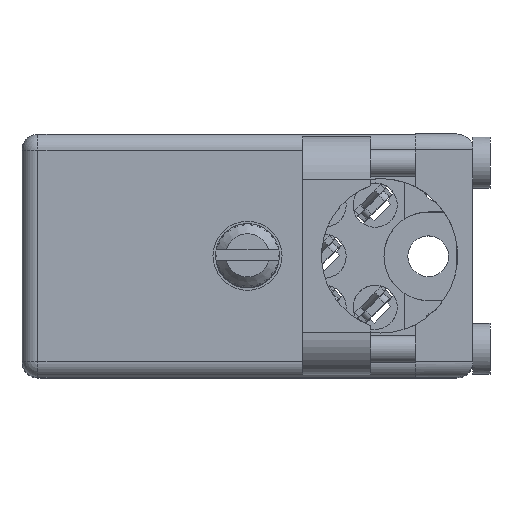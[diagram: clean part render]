
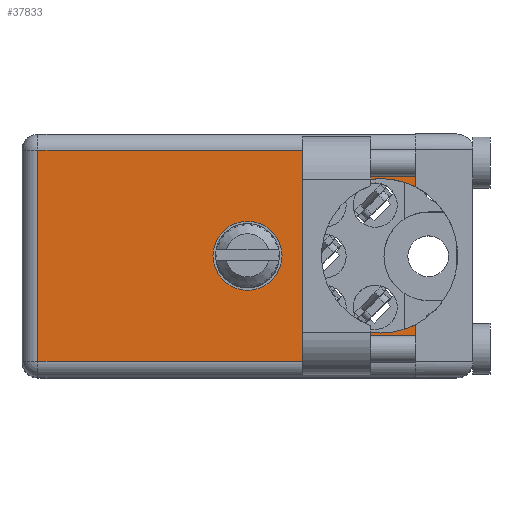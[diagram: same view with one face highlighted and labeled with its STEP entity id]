
A CAD part, top view. The second image highlights one B-rep face of the part: STEP entity #37833.
In plain terms, the highlighted face is planar.
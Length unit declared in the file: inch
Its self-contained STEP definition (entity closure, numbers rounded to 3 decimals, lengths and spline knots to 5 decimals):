
#748 = VERTEX_POINT ( 'NONE', #55095 ) ;
#920 = VERTEX_POINT ( 'NONE', #2474 ) ;
#1799 = CARTESIAN_POINT ( 'NONE',  ( 0.047, 0.906, -0.715 ) ) ;
#2474 = CARTESIAN_POINT ( 'NONE',  ( 0.047, 0.906, -0.668 ) ) ;
#3330 = CARTESIAN_POINT ( 'NONE',  ( 0.6625, 0.906, -0.256 ) ) ;
#3827 = DIRECTION ( 'NONE',  ( 0., 1., 0. ) ) ;
#4999 = DIRECTION ( 'NONE',  ( 0., 0., 1. ) ) ;
#6817 = VERTEX_POINT ( 'NONE', #141544 ) ;
#10199 = AXIS2_PLACEMENT_3D ( 'NONE', #120672, #150699, #94392 ) ;
#11066 = CARTESIAN_POINT ( 'NONE',  ( 0.6625, 0.906, -0.3575 ) ) ;
#19879 = EDGE_LOOP ( 'NONE', ( #52037, #77317, #128347, #160684, #126457, #22712, #62435, #79287 ) ) ;
#22423 = DIRECTION ( 'NONE',  ( 0., 0., 1. ) ) ;
#22712 = ORIENTED_EDGE ( 'NONE', *, *, #29579, .F. ) ;
#25193 = CARTESIAN_POINT ( 'NONE',  ( 1.053, 0.906, -0.5845 ) ) ;
#25256 = VERTEX_POINT ( 'NONE', #25193 ) ;
#26480 = EDGE_CURVE ( 'NONE', #49378, #130904, #122038, .T. ) ;
#27932 = AXIS2_PLACEMENT_3D ( 'NONE', #142008, #84781, #183186 ) ;
#29579 = EDGE_CURVE ( 'NONE', #104759, #6817, #144698, .T. ) ;
#32516 = EDGE_CURVE ( 'NONE', #6817, #130904, #122594, .T. ) ;
#33533 = CIRCLE ( 'NONE', #36447, 0.227 ) ;
#33958 = CIRCLE ( 'NONE', #27932, 0.1015 ) ;
#36340 = DIRECTION ( 'NONE',  ( 0., 0., 1. ) ) ;
#36447 = AXIS2_PLACEMENT_3D ( 'NONE', #36867, #61341, #147645 ) ;
#36867 = CARTESIAN_POINT ( 'NONE',  ( 1.053, 0.906, -0.3575 ) ) ;
#37021 = VECTOR ( 'NONE', #36340, 39.37008 ) ;
#37833 = ADVANCED_FACE ( 'NONE', ( #178746, #107539 ), #176906, .T. ) ;
#39024 = ORIENTED_EDGE ( 'NONE', *, *, #128527, .F. ) ;
#43029 = CIRCLE ( 'NONE', #64029, 0.1015 ) ;
#43716 = CIRCLE ( 'NONE', #163384, 0.227 ) ;
#45681 = EDGE_CURVE ( 'NONE', #25256, #104759, #43716, .T. ) ;
#47749 = DIRECTION ( 'NONE',  ( 0., 0., 1. ) ) ;
#48731 = DIRECTION ( 'NONE',  ( 0., 1., 0. ) ) ;
#48853 = CARTESIAN_POINT ( 'NONE',  ( 0.6625, 0.906, -0.459 ) ) ;
#49378 = VERTEX_POINT ( 'NONE', #103497 ) ;
#52037 = ORIENTED_EDGE ( 'NONE', *, *, #124893, .F. ) ;
#55095 = CARTESIAN_POINT ( 'NONE',  ( 1.155, 0.906, -0.668 ) ) ;
#56113 = DIRECTION ( 'NONE',  ( 0., 1., 0. ) ) ;
#60626 = VECTOR ( 'NONE', #92092, 39.37008 ) ;
#61341 = DIRECTION ( 'NONE',  ( 0., 1., 0. ) ) ;
#62435 = ORIENTED_EDGE ( 'NONE', *, *, #45681, .F. ) ;
#63796 = AXIS2_PLACEMENT_3D ( 'NONE', #151859, #48731, #22423 ) ;
#64029 = AXIS2_PLACEMENT_3D ( 'NONE', #11066, #56113, #125493 ) ;
#66184 = VECTOR ( 'NONE', #102685, 39.37008 ) ;
#71886 = EDGE_LOOP ( 'NONE', ( #39024, #106281 ) ) ;
#72326 = DIRECTION ( 'NONE',  ( 0., 0., 1. ) ) ;
#76281 = LINE ( 'NONE', #159812, #174469 ) ;
#77317 = ORIENTED_EDGE ( 'NONE', *, *, #85751, .T. ) ;
#79287 = ORIENTED_EDGE ( 'NONE', *, *, #99387, .F. ) ;
#84781 = DIRECTION ( 'NONE',  ( 0., 1., 0. ) ) ;
#85751 = EDGE_CURVE ( 'NONE', #748, #920, #172045, .T. ) ;
#92092 = DIRECTION ( 'NONE',  ( 1., 0., 0. ) ) ;
#94003 = CARTESIAN_POINT ( 'NONE',  ( 1.053, 0.906, -0.1305 ) ) ;
#94392 = DIRECTION ( 'NONE',  ( 0., 0., 1. ) ) ;
#97960 = VERTEX_POINT ( 'NONE', #179756 ) ;
#99387 = EDGE_CURVE ( 'NONE', #97960, #25256, #33533, .T. ) ;
#102685 = DIRECTION ( 'NONE',  ( -1., 0., 0. ) ) ;
#103497 = CARTESIAN_POINT ( 'NONE',  ( 0.047, 0.906, -0.047 ) ) ;
#104759 = VERTEX_POINT ( 'NONE', #94003 ) ;
#106281 = ORIENTED_EDGE ( 'NONE', *, *, #108848, .F. ) ;
#107539 = FACE_BOUND ( 'NONE', #71886, .T. ) ;
#108848 = EDGE_CURVE ( 'NONE', #131502, #128381, #43029, .T. ) ;
#120672 = CARTESIAN_POINT ( 'NONE',  ( 0., 0.906, -0.715 ) ) ;
#122038 = LINE ( 'NONE', #167915, #60626 ) ;
#122594 = LINE ( 'NONE', #137593, #37021 ) ;
#124397 = VECTOR ( 'NONE', #47749, 39.37008 ) ;
#124893 = EDGE_CURVE ( 'NONE', #748, #97960, #76281, .T. ) ;
#125493 = DIRECTION ( 'NONE',  ( 0., 0., 1. ) ) ;
#126457 = ORIENTED_EDGE ( 'NONE', *, *, #32516, .F. ) ;
#128347 = ORIENTED_EDGE ( 'NONE', *, *, #141928, .T. ) ;
#128381 = VERTEX_POINT ( 'NONE', #3330 ) ;
#128527 = EDGE_CURVE ( 'NONE', #128381, #131502, #33958, .T. ) ;
#130904 = VERTEX_POINT ( 'NONE', #154246 ) ;
#131409 = CARTESIAN_POINT ( 'NONE',  ( 1.053, 0.906, -0.3575 ) ) ;
#131502 = VERTEX_POINT ( 'NONE', #48853 ) ;
#137593 = CARTESIAN_POINT ( 'NONE',  ( 1.155, 0.906, 0. ) ) ;
#141544 = CARTESIAN_POINT ( 'NONE',  ( 1.155, 0.906, -0.15471 ) ) ;
#141928 = EDGE_CURVE ( 'NONE', #920, #49378, #157534, .T. ) ;
#142008 = CARTESIAN_POINT ( 'NONE',  ( 0.6625, 0.906, -0.3575 ) ) ;
#143982 = CARTESIAN_POINT ( 'NONE',  ( 0., 0.906, -0.668 ) ) ;
#144698 = CIRCLE ( 'NONE', #63796, 0.227 ) ;
#147645 = DIRECTION ( 'NONE',  ( 0., 0., 1. ) ) ;
#150699 = DIRECTION ( 'NONE',  ( 0., 1., 0. ) ) ;
#151859 = CARTESIAN_POINT ( 'NONE',  ( 1.053, 0.906, -0.3575 ) ) ;
#154246 = CARTESIAN_POINT ( 'NONE',  ( 1.155, 0.906, -0.047 ) ) ;
#157534 = LINE ( 'NONE', #1799, #124397 ) ;
#159812 = CARTESIAN_POINT ( 'NONE',  ( 1.155, 0.906, 0. ) ) ;
#160684 = ORIENTED_EDGE ( 'NONE', *, *, #26480, .T. ) ;
#163384 = AXIS2_PLACEMENT_3D ( 'NONE', #131409, #3827, #72326 ) ;
#167915 = CARTESIAN_POINT ( 'NONE',  ( 1.155, 0.906, -0.047 ) ) ;
#172045 = LINE ( 'NONE', #143982, #66184 ) ;
#174469 = VECTOR ( 'NONE', #4999, 39.37008 ) ;
#176906 = PLANE ( 'NONE',  #10199 ) ;
#178746 = FACE_OUTER_BOUND ( 'NONE', #19879, .T. ) ;
#179756 = CARTESIAN_POINT ( 'NONE',  ( 1.155, 0.906, -0.56029 ) ) ;
#183186 = DIRECTION ( 'NONE',  ( 0., 0., 1. ) ) ;
